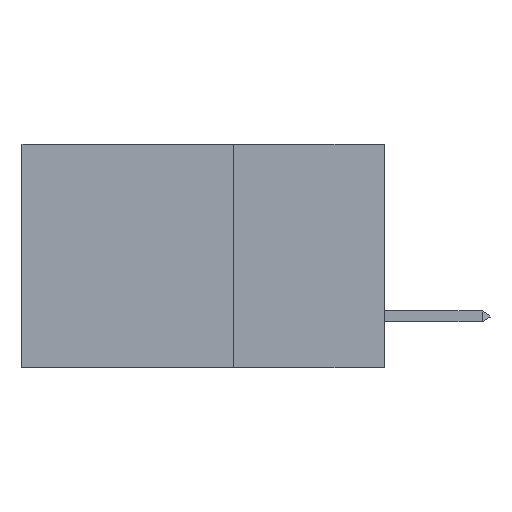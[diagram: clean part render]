
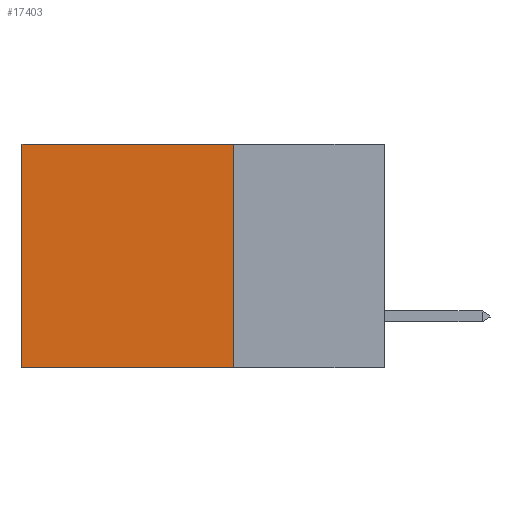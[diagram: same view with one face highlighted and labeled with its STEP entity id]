
A CAD part, left-side view. The second image highlights one B-rep face of the part: STEP entity #17403.
In plain terms, the highlighted planar face has unit normal (-1, 0, 0).
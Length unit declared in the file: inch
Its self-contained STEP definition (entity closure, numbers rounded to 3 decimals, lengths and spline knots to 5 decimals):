
#11 = DIRECTION ( 'NONE',  ( 0., 0., -1. ) ) ;
#1616 = EDGE_LOOP ( 'NONE', ( #11534, #14987, #34120, #33064 ) ) ;
#2589 = VECTOR ( 'NONE', #4925, 39.37008 ) ;
#4925 = DIRECTION ( 'NONE',  ( 0., 0., -1. ) ) ;
#5026 = EDGE_CURVE ( 'NONE', #28121, #41361, #12663, .T. ) ;
#6915 = DIRECTION ( 'NONE',  ( 0., 1., 0. ) ) ;
#7103 = EDGE_CURVE ( 'NONE', #23711, #45090, #24358, .T. ) ;
#11534 = ORIENTED_EDGE ( 'NONE', *, *, #5026, .T. ) ;
#12663 = LINE ( 'NONE', #31365, #2589 ) ;
#13431 = FACE_OUTER_BOUND ( 'NONE', #1616, .T. ) ;
#13992 = CARTESIAN_POINT ( 'NONE',  ( 0.2875, 0.25, 0. ) ) ;
#14149 = DIRECTION ( 'NONE',  ( 1., 0., 0. ) ) ;
#14987 = ORIENTED_EDGE ( 'NONE', *, *, #17284, .F. ) ;
#17284 = EDGE_CURVE ( 'NONE', #45090, #41361, #19360, .T. ) ;
#17403 = ADVANCED_FACE ( 'NONE', ( #13431 ), #33005, .F. ) ;
#19360 = LINE ( 'NONE', #43778, #48363 ) ;
#20134 = EDGE_CURVE ( 'NONE', #23711, #28121, #20849, .T. ) ;
#20849 = LINE ( 'NONE', #37000, #26159 ) ;
#21126 = DIRECTION ( 'NONE',  ( 0., 1., 0. ) ) ;
#23711 = VERTEX_POINT ( 'NONE', #31248 ) ;
#23735 = CARTESIAN_POINT ( 'NONE',  ( 0.2875, 0.25, -0.37 ) ) ;
#24358 = LINE ( 'NONE', #30243, #43294 ) ;
#26159 = VECTOR ( 'NONE', #6915, 39.37008 ) ;
#28121 = VERTEX_POINT ( 'NONE', #29693 ) ;
#29693 = CARTESIAN_POINT ( 'NONE',  ( 0.2875, 0.6, 0. ) ) ;
#30243 = CARTESIAN_POINT ( 'NONE',  ( 0.2875, 0.25, 0. ) ) ;
#31248 = CARTESIAN_POINT ( 'NONE',  ( 0.2875, 0.25, 0. ) ) ;
#31365 = CARTESIAN_POINT ( 'NONE',  ( 0.2875, 0.6, 0. ) ) ;
#33005 = PLANE ( 'NONE',  #48059 ) ;
#33064 = ORIENTED_EDGE ( 'NONE', *, *, #20134, .T. ) ;
#34120 = ORIENTED_EDGE ( 'NONE', *, *, #7103, .F. ) ;
#37000 = CARTESIAN_POINT ( 'NONE',  ( 0.2875, 0.25, 0. ) ) ;
#40623 = DIRECTION ( 'NONE',  ( 0., 0., -1. ) ) ;
#41361 = VERTEX_POINT ( 'NONE', #44385 ) ;
#43294 = VECTOR ( 'NONE', #11, 39.37008 ) ;
#43778 = CARTESIAN_POINT ( 'NONE',  ( 0.2875, 0.25, -0.37 ) ) ;
#44385 = CARTESIAN_POINT ( 'NONE',  ( 0.2875, 0.6, -0.37 ) ) ;
#45090 = VERTEX_POINT ( 'NONE', #23735 ) ;
#48059 = AXIS2_PLACEMENT_3D ( 'NONE', #13992, #14149, #40623 ) ;
#48363 = VECTOR ( 'NONE', #21126, 39.37008 ) ;
